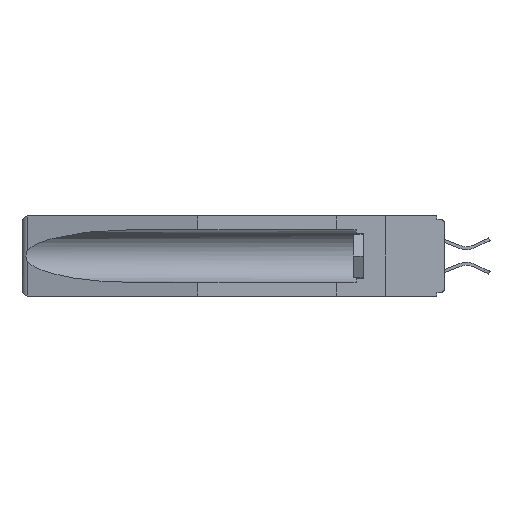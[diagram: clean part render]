
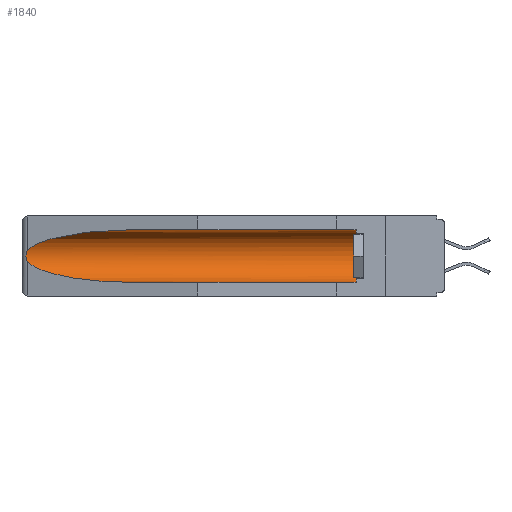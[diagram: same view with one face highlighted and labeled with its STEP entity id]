
A CAD part, left-side view. The second image highlights one B-rep face of the part: STEP entity #1840.
In plain terms, the highlighted cylindrical face has radius 2.857 mm (diameter 5.715 mm), a partial arc.
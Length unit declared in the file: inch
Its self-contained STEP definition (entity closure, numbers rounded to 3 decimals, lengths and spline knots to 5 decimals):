
#223 = EDGE_CURVE ( 'NONE', #861, #27870, #32084, .T. ) ;
#707 = CARTESIAN_POINT ( 'NONE',  ( 0.25451, 1.48313, -0.09465 ) ) ;
#821 = DIRECTION ( 'NONE',  ( 0., -1., 0. ) ) ;
#861 = VERTEX_POINT ( 'NONE', #11142 ) ;
#1743 = CARTESIAN_POINT ( 'NONE',  ( 0.2673, 1.5327, -0.16383 ) ) ;
#1840 = ADVANCED_FACE ( 'NONE', ( #21258 ), #16897, .F. ) ;
#2279 = ORIENTED_EDGE ( 'NONE', *, *, #14194, .T. ) ;
#2453 = VERTEX_POINT ( 'NONE', #3295 ) ;
#2975 = ORIENTED_EDGE ( 'NONE', *, *, #25645, .F. ) ;
#3264 = CARTESIAN_POINT ( 'NONE',  ( 0.155, -0.30754, -0.059 ) ) ;
#3295 = CARTESIAN_POINT ( 'NONE',  ( 0.26537, 1.52718, -0.19328 ) ) ;
#3726 = DIRECTION ( 'NONE',  ( 0., 1., 0. ) ) ;
#4380 = CARTESIAN_POINT ( 'NONE',  ( 0.26655, 1.53094, -0.18657 ) ) ;
#5554 =( BOUNDED_CURVE ( )  B_SPLINE_CURVE ( 3, ( #23090, #30271, #15228, #15132 ),
 .UNSPECIFIED., .F., .F. ) 
 B_SPLINE_CURVE_WITH_KNOTS ( ( 4, 4 ),
 ( 0.1948, 1.5708 ),
 .UNSPECIFIED. ) 
 CURVE ( )  GEOMETRIC_REPRESENTATION_ITEM ( )  RATIONAL_B_SPLINE_CURVE ( ( 1., 0.848, 0.848, 1. ) ) 
 REPRESENTATION_ITEM ( '' )  );
#5637 = VERTEX_POINT ( 'NONE', #23647 ) ;
#6469 = CARTESIAN_POINT ( 'NONE',  ( 0.26597, 1.5296, -0.19026 ) ) ;
#8915 = CARTESIAN_POINT ( 'NONE',  ( 0.2675, 1.53308, -0.17534 ) ) ;
#9701 = CIRCLE ( 'NONE', #19442, 0.1125 ) ;
#10009 = ORIENTED_EDGE ( 'NONE', *, *, #16200, .T. ) ;
#10567 = DIRECTION ( 'NONE',  ( 0., 1., 0. ) ) ;
#11093 = CARTESIAN_POINT ( 'NONE',  ( 0.155, 1.07973, -0.059 ) ) ;
#11142 = CARTESIAN_POINT ( 'NONE',  ( 0.155, 0.126, -0.059 ) ) ;
#11730 = CARTESIAN_POINT ( 'NONE',  ( 0.26537, 1.52718, -0.14972 ) ) ;
#11737 = CARTESIAN_POINT ( 'NONE',  ( 0.155, 0.126, -0.284 ) ) ;
#13307 = CARTESIAN_POINT ( 'NONE',  ( 0.155, 1.07973, -0.059 ) ) ;
#13533 = CARTESIAN_POINT ( 'NONE',  ( 0.26537, 1.52718, -0.14972 ) ) ;
#14157 = EDGE_CURVE ( 'NONE', #30538, #861, #9701, .T. ) ;
#14194 = EDGE_CURVE ( 'NONE', #27870, #32483, #30702, .T. ) ;
#14338 = CARTESIAN_POINT ( 'NONE',  ( 0.26654, 1.53092, -0.15636 ) ) ;
#15132 = CARTESIAN_POINT ( 'NONE',  ( 0.155, 1.07973, -0.284 ) ) ;
#15228 = CARTESIAN_POINT ( 'NONE',  ( 0.21114, 1.30732, -0.284 ) ) ;
#15298 = ORIENTED_EDGE ( 'NONE', *, *, #22148, .T. ) ;
#16200 = EDGE_CURVE ( 'NONE', #32483, #2453, #25657, .T. ) ;
#16897 = CYLINDRICAL_SURFACE ( 'NONE', #28290, 0.1125 ) ;
#19442 = AXIS2_PLACEMENT_3D ( 'NONE', #21065, #821, #25928 ) ;
#19550 = CARTESIAN_POINT ( 'NONE',  ( 0.2673, 1.53269, -0.17917 ) ) ;
#20437 = DIRECTION ( 'NONE',  ( 0., 0., 1. ) ) ;
#21065 = CARTESIAN_POINT ( 'NONE',  ( 0.155, 0.126, -0.1715 ) ) ;
#21169 = EDGE_LOOP ( 'NONE', ( #2279, #10009, #15298, #2975, #26319, #30373 ) ) ;
#21258 = FACE_OUTER_BOUND ( 'NONE', #21169, .T. ) ;
#21661 = CARTESIAN_POINT ( 'NONE',  ( 0.26597, 1.52961, -0.15275 ) ) ;
#22148 = EDGE_CURVE ( 'NONE', #2453, #5637, #5554, .T. ) ;
#22658 = CARTESIAN_POINT ( 'NONE',  ( 0.155, -0.30754, -0.1715 ) ) ;
#23090 = CARTESIAN_POINT ( 'NONE',  ( 0.26537, 1.52718, -0.19328 ) ) ;
#23418 = VECTOR ( 'NONE', #3726, 39.37008 ) ;
#23647 = CARTESIAN_POINT ( 'NONE',  ( 0.155, 1.07973, -0.284 ) ) ;
#23748 = VECTOR ( 'NONE', #10567, 39.37008 ) ;
#24070 = CARTESIAN_POINT ( 'NONE',  ( 0.26537, 1.52718, -0.19328 ) ) ;
#25645 = EDGE_CURVE ( 'NONE', #30538, #5637, #30145, .T. ) ;
#25657 = B_SPLINE_CURVE_WITH_KNOTS ( 'NONE', 3,
 ( #29481, #21661, #14338, #1743, #29166, #8915, #19550, #4380, #6469, #24070 ),
 .UNSPECIFIED., .F., .F.,
 ( 4, 2, 2, 2, 4 ),
 ( 0., 0.00029, 0.00058, 0.00087, 0.00117 ),
 .UNSPECIFIED. ) ;
#25928 = DIRECTION ( 'NONE',  ( 0., 0., 1. ) ) ;
#26319 = ORIENTED_EDGE ( 'NONE', *, *, #14157, .T. ) ;
#27870 = VERTEX_POINT ( 'NONE', #11093 ) ;
#27961 = DIRECTION ( 'NONE',  ( 0., 1., 0. ) ) ;
#28266 = CARTESIAN_POINT ( 'NONE',  ( 0.21114, 1.30732, -0.059 ) ) ;
#28290 = AXIS2_PLACEMENT_3D ( 'NONE', #22658, #27961, #20437 ) ;
#29070 = CARTESIAN_POINT ( 'NONE',  ( 0.155, -0.30754, -0.284 ) ) ;
#29166 = CARTESIAN_POINT ( 'NONE',  ( 0.2675, 1.53308, -0.16763 ) ) ;
#29481 = CARTESIAN_POINT ( 'NONE',  ( 0.26537, 1.52718, -0.14972 ) ) ;
#30145 = LINE ( 'NONE', #29070, #23418 ) ;
#30271 = CARTESIAN_POINT ( 'NONE',  ( 0.25451, 1.48313, -0.24835 ) ) ;
#30373 = ORIENTED_EDGE ( 'NONE', *, *, #223, .T. ) ;
#30538 = VERTEX_POINT ( 'NONE', #11737 ) ;
#30702 =( BOUNDED_CURVE ( )  B_SPLINE_CURVE ( 3, ( #13307, #28266, #707, #13533 ),
 .UNSPECIFIED., .F., .F. ) 
 B_SPLINE_CURVE_WITH_KNOTS ( ( 4, 4 ),
 ( 4.71239, 6.08839 ),
 .UNSPECIFIED. ) 
 CURVE ( )  GEOMETRIC_REPRESENTATION_ITEM ( )  RATIONAL_B_SPLINE_CURVE ( ( 1., 0.848, 0.848, 1. ) ) 
 REPRESENTATION_ITEM ( '' )  );
#32084 = LINE ( 'NONE', #3264, #23748 ) ;
#32483 = VERTEX_POINT ( 'NONE', #11730 ) ;
